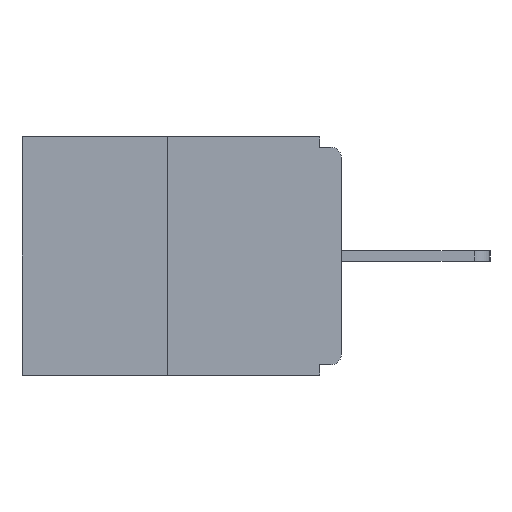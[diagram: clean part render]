
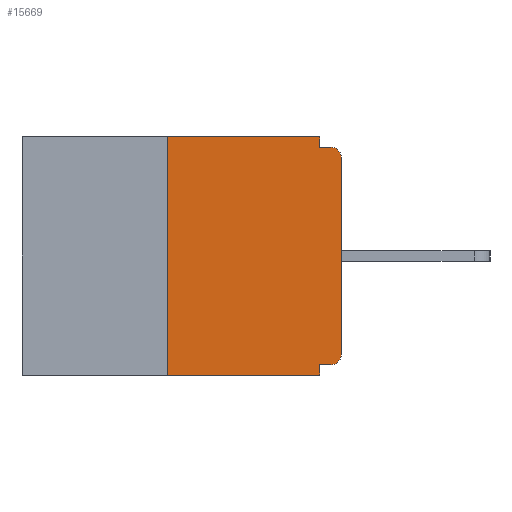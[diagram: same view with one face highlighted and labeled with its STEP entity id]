
A CAD part, left-side view. The second image highlights one B-rep face of the part: STEP entity #15669.
In plain terms, the highlighted planar face has unit normal (-1, 0, 0).
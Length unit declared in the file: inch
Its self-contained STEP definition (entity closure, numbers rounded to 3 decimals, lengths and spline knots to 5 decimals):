
#289 = DIRECTION ( 'NONE',  ( 0., 0., 1. ) ) ;
#956 = VERTEX_POINT ( 'NONE', #5464 ) ;
#2039 = LINE ( 'NONE', #15646, #21771 ) ;
#2179 = EDGE_CURVE ( 'NONE', #21020, #7819, #3180, .T. ) ;
#2334 = LINE ( 'NONE', #20282, #4138 ) ;
#2826 = ORIENTED_EDGE ( 'NONE', *, *, #16145, .T. ) ;
#2932 = EDGE_CURVE ( 'NONE', #5782, #12340, #5310, .T. ) ;
#3180 = LINE ( 'NONE', #24914, #20117 ) ;
#3390 = CARTESIAN_POINT ( 'NONE',  ( 0., 0.015, -0.313 ) ) ;
#3951 = VECTOR ( 'NONE', #14650, 39.37008 ) ;
#4138 = VECTOR ( 'NONE', #8212, 39.37008 ) ;
#4175 = EDGE_CURVE ( 'NONE', #5065, #11504, #18798, .T. ) ;
#4305 = ORIENTED_EDGE ( 'NONE', *, *, #22854, .T. ) ;
#4968 = DIRECTION ( 'NONE',  ( 0., 0., -1. ) ) ;
#5065 = VERTEX_POINT ( 'NONE', #20296 ) ;
#5251 = EDGE_CURVE ( 'NONE', #13676, #956, #24466, .T. ) ;
#5310 = LINE ( 'NONE', #21035, #22794 ) ;
#5464 = CARTESIAN_POINT ( 'NONE',  ( 0., 0.031, 0. ) ) ;
#5782 = VERTEX_POINT ( 'NONE', #21765 ) ;
#5816 = DIRECTION ( 'NONE',  ( -1., 0., 0. ) ) ;
#5879 = VECTOR ( 'NONE', #289, 39.37008 ) ;
#6195 = ORIENTED_EDGE ( 'NONE', *, *, #5251, .F. ) ;
#6460 = ORIENTED_EDGE ( 'NONE', *, *, #2179, .F. ) ;
#6671 = VECTOR ( 'NONE', #17605, 39.37008 ) ;
#6878 = CARTESIAN_POINT ( 'NONE',  ( 0., 0.031, -0.328 ) ) ;
#6907 = CARTESIAN_POINT ( 'NONE',  ( 0., 0.46, 0. ) ) ;
#6924 = CARTESIAN_POINT ( 'NONE',  ( 0., 0.46, 0. ) ) ;
#7300 = EDGE_LOOP ( 'NONE', ( #6195, #12613, #11585, #6460, #20594, #13542, #4305, #2826, #9451, #11047 ) ) ;
#7523 = AXIS2_PLACEMENT_3D ( 'NONE', #3390, #14897, #4968 ) ;
#7584 = CARTESIAN_POINT ( 'NONE',  ( 0., 0., -0.03 ) ) ;
#7672 = DIRECTION ( 'NONE',  ( 1., 0., 0. ) ) ;
#7819 = VERTEX_POINT ( 'NONE', #15460 ) ;
#8212 = DIRECTION ( 'NONE',  ( 0., -1., 0. ) ) ;
#9412 = LINE ( 'NONE', #17417, #24013 ) ;
#9451 = ORIENTED_EDGE ( 'NONE', *, *, #2932, .F. ) ;
#10210 = CARTESIAN_POINT ( 'NONE',  ( 0., 0.25, 0. ) ) ;
#11047 = ORIENTED_EDGE ( 'NONE', *, *, #17760, .F. ) ;
#11164 = EDGE_CURVE ( 'NONE', #5065, #21020, #9412, .T. ) ;
#11504 = VERTEX_POINT ( 'NONE', #11897 ) ;
#11585 = ORIENTED_EDGE ( 'NONE', *, *, #15450, .T. ) ;
#11897 = CARTESIAN_POINT ( 'NONE',  ( 0., 0., -0.313 ) ) ;
#12340 = VERTEX_POINT ( 'NONE', #18712 ) ;
#12613 = ORIENTED_EDGE ( 'NONE', *, *, #18355, .F. ) ;
#12886 = AXIS2_PLACEMENT_3D ( 'NONE', #25604, #5816, #13807 ) ;
#12904 = CIRCLE ( 'NONE', #12886, 0.015 ) ;
#13308 = CARTESIAN_POINT ( 'NONE',  ( 0., 0.031, 0. ) ) ;
#13542 = ORIENTED_EDGE ( 'NONE', *, *, #4175, .T. ) ;
#13676 = VERTEX_POINT ( 'NONE', #23967 ) ;
#13807 = DIRECTION ( 'NONE',  ( 0., 0., -1. ) ) ;
#14171 = VERTEX_POINT ( 'NONE', #20914 ) ;
#14650 = DIRECTION ( 'NONE',  ( 0., -1., 0. ) ) ;
#14897 = DIRECTION ( 'NONE',  ( -1., 0., 0. ) ) ;
#15088 = DIRECTION ( 'NONE',  ( 0., 0., -1. ) ) ;
#15254 = LINE ( 'NONE', #13308, #6671 ) ;
#15375 = VERTEX_POINT ( 'NONE', #7584 ) ;
#15450 = EDGE_CURVE ( 'NONE', #14171, #7819, #2334, .T. ) ;
#15460 = CARTESIAN_POINT ( 'NONE',  ( 0., 0.031, -0.343 ) ) ;
#15646 = CARTESIAN_POINT ( 'NONE',  ( 0., 0., 0. ) ) ;
#15669 = ADVANCED_FACE ( 'NONE', ( #21179 ), #18807, .F. ) ;
#16145 = EDGE_CURVE ( 'NONE', #15375, #12340, #12904, .T. ) ;
#17417 = CARTESIAN_POINT ( 'NONE',  ( 0., 0., -0.328 ) ) ;
#17605 = DIRECTION ( 'NONE',  ( 0., 0., -1. ) ) ;
#17760 = EDGE_CURVE ( 'NONE', #956, #5782, #15254, .T. ) ;
#18355 = EDGE_CURVE ( 'NONE', #14171, #13676, #20329, .T. ) ;
#18712 = CARTESIAN_POINT ( 'NONE',  ( 0., 0.015, -0.015 ) ) ;
#18798 = CIRCLE ( 'NONE', #7523, 0.015 ) ;
#18807 = PLANE ( 'NONE',  #24201 ) ;
#20117 = VECTOR ( 'NONE', #15088, 39.37008 ) ;
#20282 = CARTESIAN_POINT ( 'NONE',  ( 0., 0.46, -0.343 ) ) ;
#20296 = CARTESIAN_POINT ( 'NONE',  ( 0., 0.015, -0.328 ) ) ;
#20329 = LINE ( 'NONE', #10210, #5879 ) ;
#20594 = ORIENTED_EDGE ( 'NONE', *, *, #11164, .F. ) ;
#20914 = CARTESIAN_POINT ( 'NONE',  ( 0., 0.25, -0.343 ) ) ;
#21020 = VERTEX_POINT ( 'NONE', #6878 ) ;
#21035 = CARTESIAN_POINT ( 'NONE',  ( 0., 0., -0.015 ) ) ;
#21179 = FACE_OUTER_BOUND ( 'NONE', #7300, .T. ) ;
#21426 = DIRECTION ( 'NONE',  ( 0., -1., 0. ) ) ;
#21765 = CARTESIAN_POINT ( 'NONE',  ( 0., 0.031, -0.015 ) ) ;
#21771 = VECTOR ( 'NONE', #25873, 39.37008 ) ;
#22794 = VECTOR ( 'NONE', #21426, 39.37008 ) ;
#22854 = EDGE_CURVE ( 'NONE', #11504, #15375, #2039, .T. ) ;
#23655 = DIRECTION ( 'NONE',  ( 0., 0., -1. ) ) ;
#23967 = CARTESIAN_POINT ( 'NONE',  ( 0., 0.25, 0. ) ) ;
#24013 = VECTOR ( 'NONE', #25418, 39.37008 ) ;
#24201 = AXIS2_PLACEMENT_3D ( 'NONE', #6907, #7672, #23655 ) ;
#24466 = LINE ( 'NONE', #6924, #3951 ) ;
#24914 = CARTESIAN_POINT ( 'NONE',  ( 0., 0.031, -0.343 ) ) ;
#25418 = DIRECTION ( 'NONE',  ( 0., 1., 0. ) ) ;
#25604 = CARTESIAN_POINT ( 'NONE',  ( 0., 0.015, -0.03 ) ) ;
#25873 = DIRECTION ( 'NONE',  ( 0., 0., 1. ) ) ;
